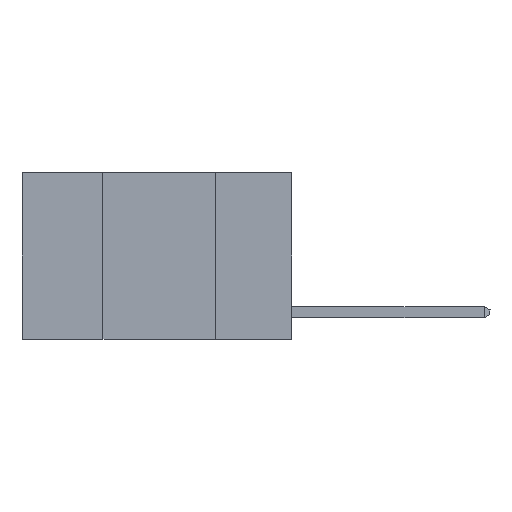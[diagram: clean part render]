
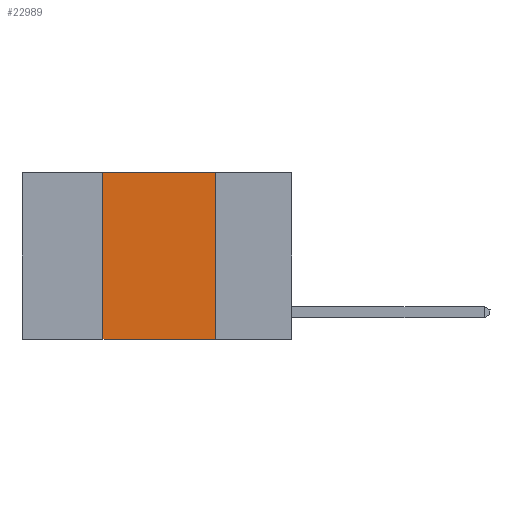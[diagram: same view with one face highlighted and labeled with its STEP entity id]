
A CAD part, left-side view. The second image highlights one B-rep face of the part: STEP entity #22989.
In plain terms, the highlighted planar face has unit normal (-1, 0, 0).
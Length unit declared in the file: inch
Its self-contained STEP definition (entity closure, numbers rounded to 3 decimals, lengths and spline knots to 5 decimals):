
#466 = DIRECTION ( 'NONE',  ( 0., 0., -1. ) ) ;
#487 = EDGE_CURVE ( 'NONE', #16446, #12716, #2371, .T. ) ;
#2371 = LINE ( 'NONE', #11418, #7232 ) ;
#2974 = ORIENTED_EDGE ( 'NONE', *, *, #4682, .F. ) ;
#4456 = EDGE_CURVE ( 'NONE', #17498, #18210, #25572, .T. ) ;
#4682 = EDGE_CURVE ( 'NONE', #16446, #17498, #9474, .T. ) ;
#4972 = VECTOR ( 'NONE', #25777, 39.37008 ) ;
#5761 = CARTESIAN_POINT ( 'NONE',  ( 0., 0.17, -0.37 ) ) ;
#7232 = VECTOR ( 'NONE', #16602, 39.37008 ) ;
#7435 = EDGE_CURVE ( 'NONE', #18210, #12716, #17031, .T. ) ;
#9202 = CARTESIAN_POINT ( 'NONE',  ( 0., 0.42, 0. ) ) ;
#9474 = LINE ( 'NONE', #26370, #19790 ) ;
#9636 = EDGE_LOOP ( 'NONE', ( #22949, #18745, #2974, #13847 ) ) ;
#10777 = CARTESIAN_POINT ( 'NONE',  ( 0., 0.6, 0. ) ) ;
#11418 = CARTESIAN_POINT ( 'NONE',  ( 0., 0.6, -0.37 ) ) ;
#11826 = DIRECTION ( 'NONE',  ( 0., 0., -1. ) ) ;
#12716 = VERTEX_POINT ( 'NONE', #5761 ) ;
#12844 = DIRECTION ( 'NONE',  ( 1., 0., 0. ) ) ;
#13446 = CARTESIAN_POINT ( 'NONE',  ( 0., 0.6, 0. ) ) ;
#13847 = ORIENTED_EDGE ( 'NONE', *, *, #487, .T. ) ;
#14242 = CARTESIAN_POINT ( 'NONE',  ( 0., 0.42, -0.37 ) ) ;
#16446 = VERTEX_POINT ( 'NONE', #14242 ) ;
#16602 = DIRECTION ( 'NONE',  ( 0., -1., 0. ) ) ;
#16891 = PLANE ( 'NONE',  #25809 ) ;
#17031 = LINE ( 'NONE', #22120, #17699 ) ;
#17498 = VERTEX_POINT ( 'NONE', #9202 ) ;
#17699 = VECTOR ( 'NONE', #11826, 39.37008 ) ;
#18210 = VERTEX_POINT ( 'NONE', #24829 ) ;
#18745 = ORIENTED_EDGE ( 'NONE', *, *, #4456, .F. ) ;
#19790 = VECTOR ( 'NONE', #26454, 39.37008 ) ;
#20840 = FACE_OUTER_BOUND ( 'NONE', #9636, .T. ) ;
#22120 = CARTESIAN_POINT ( 'NONE',  ( 0., 0.17, 0. ) ) ;
#22949 = ORIENTED_EDGE ( 'NONE', *, *, #7435, .F. ) ;
#22989 = ADVANCED_FACE ( 'NONE', ( #20840 ), #16891, .F. ) ;
#24829 = CARTESIAN_POINT ( 'NONE',  ( 0., 0.17, 0. ) ) ;
#25572 = LINE ( 'NONE', #13446, #4972 ) ;
#25777 = DIRECTION ( 'NONE',  ( 0., -1., 0. ) ) ;
#25809 = AXIS2_PLACEMENT_3D ( 'NONE', #10777, #12844, #466 ) ;
#26370 = CARTESIAN_POINT ( 'NONE',  ( 0., 0.42, 0. ) ) ;
#26454 = DIRECTION ( 'NONE',  ( 0., 0., 1. ) ) ;
